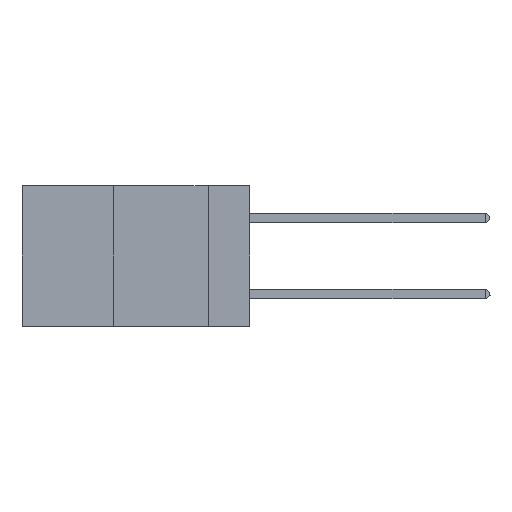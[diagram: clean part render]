
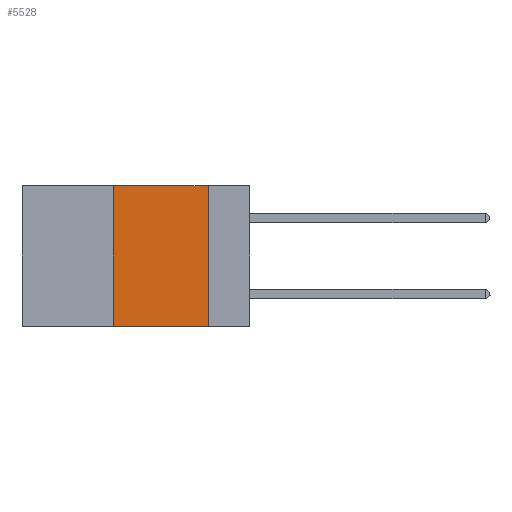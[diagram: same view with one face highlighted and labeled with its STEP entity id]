
A CAD part, left-side view. The second image highlights one B-rep face of the part: STEP entity #5528.
In plain terms, the highlighted planar face has unit normal (-1, 0, 0).
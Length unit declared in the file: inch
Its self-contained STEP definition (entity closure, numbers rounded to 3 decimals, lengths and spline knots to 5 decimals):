
#83 = DIRECTION ( 'NONE',  ( 0., 0., 1. ) ) ;
#984 = LINE ( 'NONE', #11101, #3779 ) ;
#1217 = LINE ( 'NONE', #1582, #4602 ) ;
#1582 = CARTESIAN_POINT ( 'NONE',  ( 0., 0.6, -0.37 ) ) ;
#1685 = CARTESIAN_POINT ( 'NONE',  ( 0., 0.36, 0. ) ) ;
#1822 = ORIENTED_EDGE ( 'NONE', *, *, #14476, .T. ) ;
#2095 = VECTOR ( 'NONE', #6884, 39.37008 ) ;
#2526 = CARTESIAN_POINT ( 'NONE',  ( 0., 0.11, 0. ) ) ;
#2877 = EDGE_CURVE ( 'NONE', #2931, #4919, #984, .T. ) ;
#2931 = VERTEX_POINT ( 'NONE', #2526 ) ;
#3334 = CARTESIAN_POINT ( 'NONE',  ( 0., 0.6, 0. ) ) ;
#3610 = CARTESIAN_POINT ( 'NONE',  ( 0., 0.36, 0. ) ) ;
#3631 = EDGE_CURVE ( 'NONE', #12626, #2931, #9242, .T. ) ;
#3779 = VECTOR ( 'NONE', #5060, 39.37008 ) ;
#3786 = EDGE_CURVE ( 'NONE', #15542, #12626, #7348, .T. ) ;
#4113 = AXIS2_PLACEMENT_3D ( 'NONE', #7786, #8865, #4198 ) ;
#4198 = DIRECTION ( 'NONE',  ( 0., 0., -1. ) ) ;
#4602 = VECTOR ( 'NONE', #6462, 39.37008 ) ;
#4760 = ORIENTED_EDGE ( 'NONE', *, *, #3631, .F. ) ;
#4919 = VERTEX_POINT ( 'NONE', #5159 ) ;
#5060 = DIRECTION ( 'NONE',  ( 0., 0., -1. ) ) ;
#5159 = CARTESIAN_POINT ( 'NONE',  ( 0., 0.11, -0.37 ) ) ;
#5528 = ADVANCED_FACE ( 'NONE', ( #5821 ), #7732, .F. ) ;
#5821 = FACE_OUTER_BOUND ( 'NONE', #6338, .T. ) ;
#6338 = EDGE_LOOP ( 'NONE', ( #10700, #4760, #11299, #1822 ) ) ;
#6462 = DIRECTION ( 'NONE',  ( 0., -1., 0. ) ) ;
#6884 = DIRECTION ( 'NONE',  ( 0., -1., 0. ) ) ;
#7348 = LINE ( 'NONE', #1685, #14823 ) ;
#7732 = PLANE ( 'NONE',  #4113 ) ;
#7786 = CARTESIAN_POINT ( 'NONE',  ( 0., 0.6, 0. ) ) ;
#8865 = DIRECTION ( 'NONE',  ( 1., 0., 0. ) ) ;
#9242 = LINE ( 'NONE', #3334, #2095 ) ;
#10700 = ORIENTED_EDGE ( 'NONE', *, *, #2877, .F. ) ;
#11101 = CARTESIAN_POINT ( 'NONE',  ( 0., 0.11, 0. ) ) ;
#11299 = ORIENTED_EDGE ( 'NONE', *, *, #3786, .F. ) ;
#12626 = VERTEX_POINT ( 'NONE', #3610 ) ;
#14476 = EDGE_CURVE ( 'NONE', #15542, #4919, #1217, .T. ) ;
#14616 = CARTESIAN_POINT ( 'NONE',  ( 0., 0.36, -0.37 ) ) ;
#14823 = VECTOR ( 'NONE', #83, 39.37008 ) ;
#15542 = VERTEX_POINT ( 'NONE', #14616 ) ;
